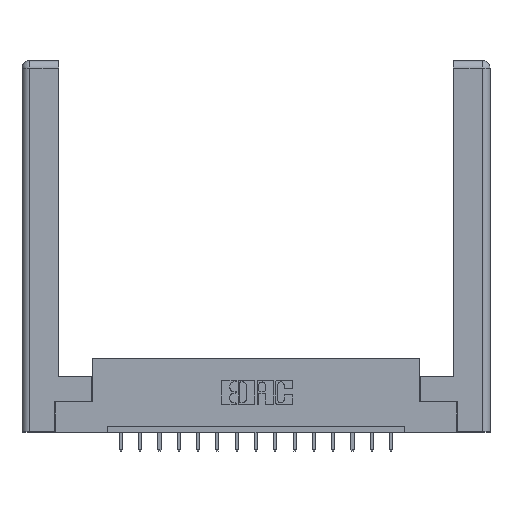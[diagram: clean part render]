
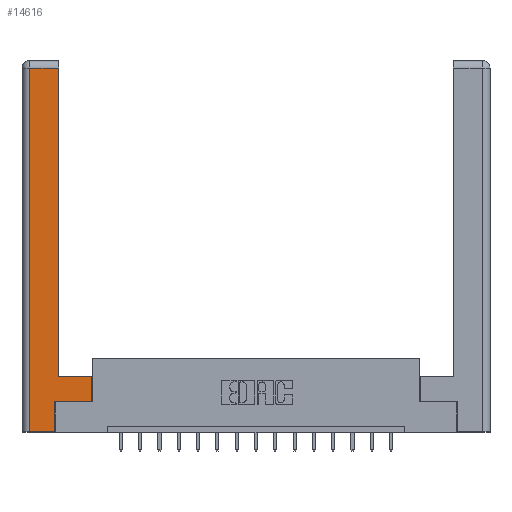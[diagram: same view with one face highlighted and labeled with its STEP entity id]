
A CAD part, top view. The second image highlights one B-rep face of the part: STEP entity #14616.
In plain terms, the highlighted planar face has unit normal (0, 0, 1).
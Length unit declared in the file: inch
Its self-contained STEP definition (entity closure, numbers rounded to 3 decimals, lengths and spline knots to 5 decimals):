
#131 = VECTOR ( 'NONE', #16390, 39.37008 ) ;
#458 = EDGE_CURVE ( 'NONE', #15549, #9295, #8496, .T. ) ;
#520 = VERTEX_POINT ( 'NONE', #9193 ) ;
#697 = LINE ( 'NONE', #6847, #14056 ) ;
#807 = VECTOR ( 'NONE', #13195, 39.37008 ) ;
#826 = VERTEX_POINT ( 'NONE', #15404 ) ;
#1112 = CARTESIAN_POINT ( 'NONE',  ( 0.565, 0.45, 0. ) ) ;
#1134 = CARTESIAN_POINT ( 'NONE',  ( 0.0615, 0., 0. ) ) ;
#1161 = LINE ( 'NONE', #7316, #7414 ) ;
#1399 = DIRECTION ( 'NONE',  ( 1., 0., 0. ) ) ;
#1510 = VECTOR ( 'NONE', #6784, 39.37008 ) ;
#2088 = ORIENTED_EDGE ( 'NONE', *, *, #7875, .T. ) ;
#2754 = ORIENTED_EDGE ( 'NONE', *, *, #12135, .T. ) ;
#3841 = EDGE_CURVE ( 'NONE', #14759, #826, #10217, .T. ) ;
#4217 = ORIENTED_EDGE ( 'NONE', *, *, #16022, .T. ) ;
#4991 = VECTOR ( 'NONE', #14542, 39.37008 ) ;
#5177 = CARTESIAN_POINT ( 'NONE',  ( 0.265, 0.245, 0. ) ) ;
#5272 = DIRECTION ( 'NONE',  ( -1., 0., 0. ) ) ;
#5678 = CARTESIAN_POINT ( 'NONE',  ( 0.565, 0.245, 0. ) ) ;
#5951 = LINE ( 'NONE', #8361, #131 ) ;
#6572 = PLANE ( 'NONE',  #13990 ) ;
#6784 = DIRECTION ( 'NONE',  ( 1., 0., 0. ) ) ;
#6847 = CARTESIAN_POINT ( 'NONE',  ( 0.265, 0., 0. ) ) ;
#7316 = CARTESIAN_POINT ( 'NONE',  ( 0.295, 0.45, 0. ) ) ;
#7414 = VECTOR ( 'NONE', #8614, 39.37008 ) ;
#7683 = CARTESIAN_POINT ( 'NONE',  ( 0.0615, 2.94, 0. ) ) ;
#7856 = ORIENTED_EDGE ( 'NONE', *, *, #15322, .T. ) ;
#7875 = EDGE_CURVE ( 'NONE', #520, #14759, #8410, .T. ) ;
#7931 = ORIENTED_EDGE ( 'NONE', *, *, #9737, .T. ) ;
#8361 = CARTESIAN_POINT ( 'NONE',  ( 0.295, 3., 0. ) ) ;
#8410 = LINE ( 'NONE', #14777, #1510 ) ;
#8496 = LINE ( 'NONE', #1134, #13896 ) ;
#8505 = ORIENTED_EDGE ( 'NONE', *, *, #458, .T. ) ;
#8553 = EDGE_CURVE ( 'NONE', #9694, #15549, #11942, .T. ) ;
#8614 = DIRECTION ( 'NONE',  ( -1., 0., 0. ) ) ;
#9193 = CARTESIAN_POINT ( 'NONE',  ( 0.265, 0.245, 0. ) ) ;
#9295 = VERTEX_POINT ( 'NONE', #9839 ) ;
#9316 = DIRECTION ( 'NONE',  ( 0., -1., 0. ) ) ;
#9694 = VERTEX_POINT ( 'NONE', #14720 ) ;
#9737 = EDGE_CURVE ( 'NONE', #9295, #16208, #697, .T. ) ;
#9839 = CARTESIAN_POINT ( 'NONE',  ( 0.0615, 0., 0. ) ) ;
#10217 = LINE ( 'NONE', #1112, #807 ) ;
#11936 = CARTESIAN_POINT ( 'NONE',  ( 0., 0., 0. ) ) ;
#11942 = LINE ( 'NONE', #7683, #15274 ) ;
#12132 = LINE ( 'NONE', #5177, #4991 ) ;
#12135 = EDGE_CURVE ( 'NONE', #16208, #520, #12132, .T. ) ;
#13195 = DIRECTION ( 'NONE',  ( 0., 1., 0. ) ) ;
#13284 = DIRECTION ( 'NONE',  ( 0., 0., -1. ) ) ;
#13419 = ORIENTED_EDGE ( 'NONE', *, *, #3841, .T. ) ;
#13526 = CARTESIAN_POINT ( 'NONE',  ( 0.295, 0.45, 0. ) ) ;
#13710 = FACE_OUTER_BOUND ( 'NONE', #16957, .T. ) ;
#13896 = VECTOR ( 'NONE', #9316, 39.37008 ) ;
#13990 = AXIS2_PLACEMENT_3D ( 'NONE', #11936, #13284, #5272 ) ;
#14056 = VECTOR ( 'NONE', #1399, 39.37008 ) ;
#14542 = DIRECTION ( 'NONE',  ( 0., 1., 0. ) ) ;
#14616 = ADVANCED_FACE ( 'NONE', ( #13710 ), #6572, .F. ) ;
#14720 = CARTESIAN_POINT ( 'NONE',  ( 0.295, 2.94, 0. ) ) ;
#14759 = VERTEX_POINT ( 'NONE', #5678 ) ;
#14777 = CARTESIAN_POINT ( 'NONE',  ( 0.565, 0.245, 0. ) ) ;
#15195 = VERTEX_POINT ( 'NONE', #13526 ) ;
#15274 = VECTOR ( 'NONE', #15789, 39.37008 ) ;
#15322 = EDGE_CURVE ( 'NONE', #15195, #9694, #5951, .T. ) ;
#15354 = CARTESIAN_POINT ( 'NONE',  ( 0.265, 0., 0. ) ) ;
#15404 = CARTESIAN_POINT ( 'NONE',  ( 0.565, 0.45, 0. ) ) ;
#15549 = VERTEX_POINT ( 'NONE', #17083 ) ;
#15789 = DIRECTION ( 'NONE',  ( -1., 0., 0. ) ) ;
#16022 = EDGE_CURVE ( 'NONE', #826, #15195, #1161, .T. ) ;
#16208 = VERTEX_POINT ( 'NONE', #15354 ) ;
#16390 = DIRECTION ( 'NONE',  ( 0., 1., 0. ) ) ;
#16672 = ORIENTED_EDGE ( 'NONE', *, *, #8553, .T. ) ;
#16957 = EDGE_LOOP ( 'NONE', ( #7856, #16672, #8505, #7931, #2754, #2088, #13419, #4217 ) ) ;
#17083 = CARTESIAN_POINT ( 'NONE',  ( 0.0615, 2.94, 0. ) ) ;
